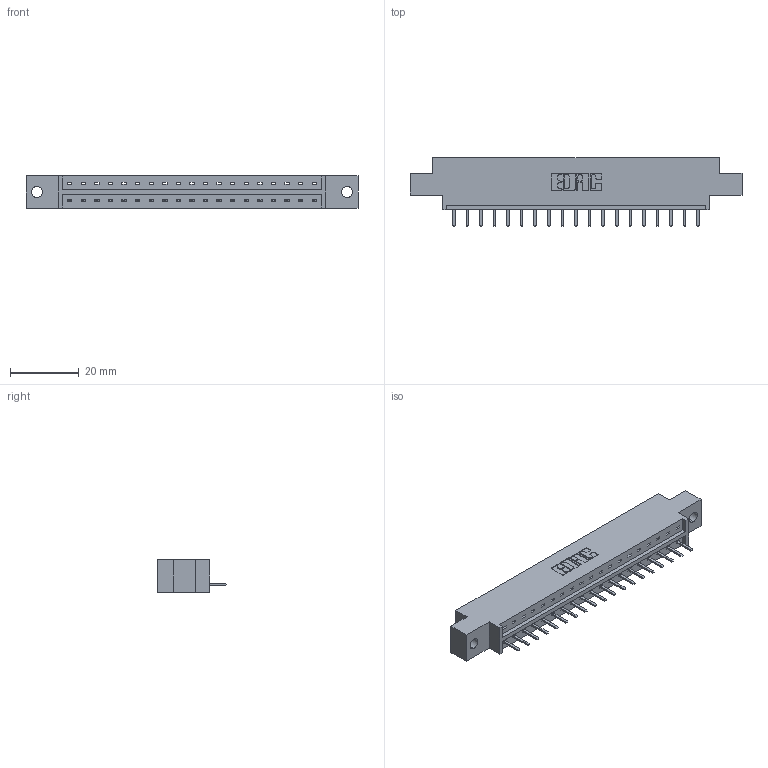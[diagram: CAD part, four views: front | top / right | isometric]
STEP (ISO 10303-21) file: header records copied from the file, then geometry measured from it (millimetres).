
FILE_DESCRIPTION (( 'STEP AP203' ), '1' );
FILE_NAME ('833-019-520-602.STEP', '2020-05-31T23:57:00', ( '' ), ( '' ), 'SwSTEP 2.0', 'SolidWorks 2020', '' );
FILE_SCHEMA (( 'CONFIG_CONTROL_DESIGN' ));
Length unit declared in the file: inch
Products named in the file (3): 833-019-520-602; 833 Part_Offset - .128 Dia; 345-292-001_345-293-120
Assembly tree (20 placements, depth 2):
  833-019-520-602
    833 Part_Offset - .128 Dia
    345-292-001_345-293-120  x19
Bounding box: 96.82 x 20.02 x 9.4 mm (x, y, z)
Volume: 9226.4 mm3; surface area: 9566.2 mm2
Topology: 20 solids, 20 shells, 1296 faces, 3819 edges, 2494 vertices
Faces by surface type: plane 910, cylinder 386
Entity records: 14839 total; most frequent: CARTESIAN_POINT 2583, ORIENTED_EDGE 2526, DIRECTION 2213, EDGE_CURVE 1263, VECTOR 1131, LINE 1131, VERTEX_POINT 838, AXIS2_PLACEMENT_3D 541
